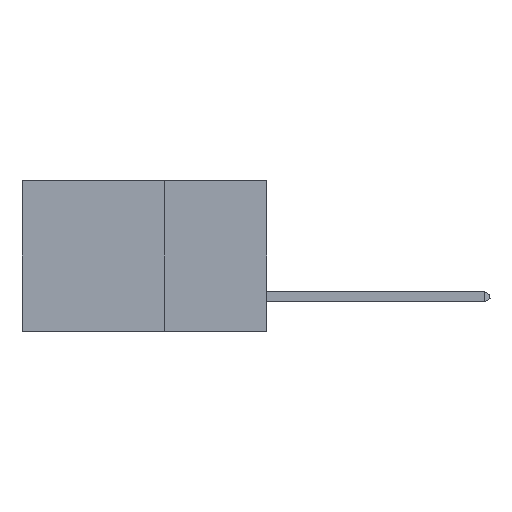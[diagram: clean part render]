
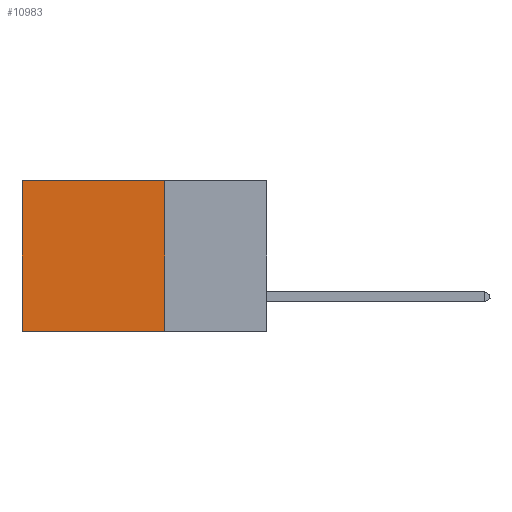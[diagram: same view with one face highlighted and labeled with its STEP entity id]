
A CAD part, left-side view. The second image highlights one B-rep face of the part: STEP entity #10983.
In plain terms, the highlighted planar face has unit normal (-1, 0, 0).
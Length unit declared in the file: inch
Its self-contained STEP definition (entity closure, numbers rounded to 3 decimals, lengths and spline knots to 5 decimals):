
#917 = PLANE ( 'NONE',  #29307 ) ;
#1212 = ORIENTED_EDGE ( 'NONE', *, *, #2670, .T. ) ;
#2670 = EDGE_CURVE ( 'NONE', #28257, #31798, #23862, .T. ) ;
#4362 = CARTESIAN_POINT ( 'NONE',  ( 0.2875, 0.6, 0. ) ) ;
#4720 = DIRECTION ( 'NONE',  ( 0., 0., -1. ) ) ;
#5988 = ORIENTED_EDGE ( 'NONE', *, *, #18234, .F. ) ;
#6368 = VECTOR ( 'NONE', #4720, 39.37008 ) ;
#7739 = VERTEX_POINT ( 'NONE', #8491 ) ;
#7756 = CARTESIAN_POINT ( 'NONE',  ( 0.2875, 0.25, 0. ) ) ;
#8035 = CARTESIAN_POINT ( 'NONE',  ( 0.2875, 0.25, 0. ) ) ;
#8491 = CARTESIAN_POINT ( 'NONE',  ( 0.2875, 0.6, -0.37 ) ) ;
#8702 = VERTEX_POINT ( 'NONE', #17104 ) ;
#9203 = EDGE_CURVE ( 'NONE', #31798, #7739, #9835, .T. ) ;
#9835 = LINE ( 'NONE', #15970, #17030 ) ;
#10473 = LINE ( 'NONE', #7756, #6368 ) ;
#10983 = ADVANCED_FACE ( 'NONE', ( #26915 ), #917, .F. ) ;
#13581 = DIRECTION ( 'NONE',  ( 0., 0., -1. ) ) ;
#14452 = DIRECTION ( 'NONE',  ( 1., 0., 0. ) ) ;
#15970 = CARTESIAN_POINT ( 'NONE',  ( 0.2875, 0.6, 0. ) ) ;
#17030 = VECTOR ( 'NONE', #18837, 39.37008 ) ;
#17104 = CARTESIAN_POINT ( 'NONE',  ( 0.2875, 0.25, -0.37 ) ) ;
#17315 = EDGE_LOOP ( 'NONE', ( #18674, #5988, #24780, #1212 ) ) ;
#18234 = EDGE_CURVE ( 'NONE', #8702, #7739, #36986, .T. ) ;
#18674 = ORIENTED_EDGE ( 'NONE', *, *, #9203, .T. ) ;
#18837 = DIRECTION ( 'NONE',  ( 0., 0., -1. ) ) ;
#19002 = EDGE_CURVE ( 'NONE', #28257, #8702, #10473, .T. ) ;
#20346 = DIRECTION ( 'NONE',  ( 0., 1., 0. ) ) ;
#23615 = CARTESIAN_POINT ( 'NONE',  ( 0.2875, 0.25, 0. ) ) ;
#23862 = LINE ( 'NONE', #23615, #23911 ) ;
#23911 = VECTOR ( 'NONE', #30930, 39.37008 ) ;
#24780 = ORIENTED_EDGE ( 'NONE', *, *, #19002, .F. ) ;
#26915 = FACE_OUTER_BOUND ( 'NONE', #17315, .T. ) ;
#28160 = CARTESIAN_POINT ( 'NONE',  ( 0.2875, 0.25, -0.37 ) ) ;
#28257 = VERTEX_POINT ( 'NONE', #8035 ) ;
#29307 = AXIS2_PLACEMENT_3D ( 'NONE', #30747, #14452, #13581 ) ;
#30747 = CARTESIAN_POINT ( 'NONE',  ( 0.2875, 0.25, 0. ) ) ;
#30930 = DIRECTION ( 'NONE',  ( 0., 1., 0. ) ) ;
#31798 = VERTEX_POINT ( 'NONE', #4362 ) ;
#36074 = VECTOR ( 'NONE', #20346, 39.37008 ) ;
#36986 = LINE ( 'NONE', #28160, #36074 ) ;
